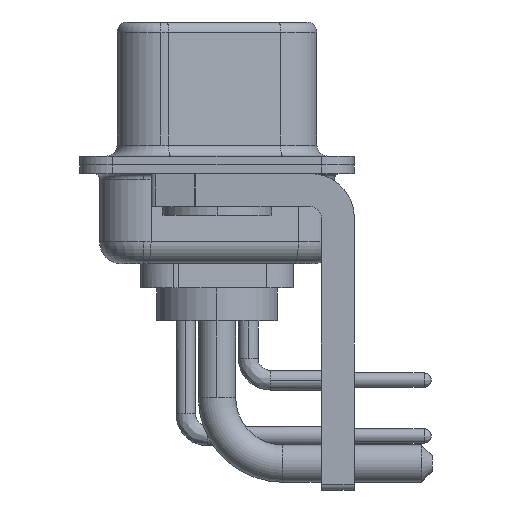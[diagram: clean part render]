
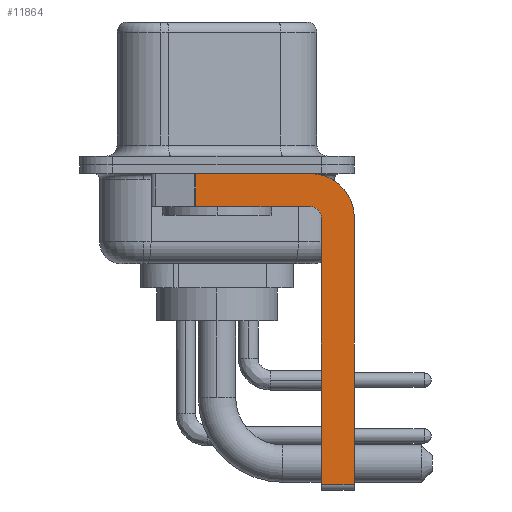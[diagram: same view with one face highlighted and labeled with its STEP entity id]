
A CAD part, left-side view. The second image highlights one B-rep face of the part: STEP entity #11864.
In plain terms, the highlighted planar face has unit normal (-1, 0, 0).
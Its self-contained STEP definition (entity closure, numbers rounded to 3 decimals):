
#256 = EDGE_CURVE ( 'NONE', #3288, #9810, #10729, .T. ) ;
#494 = DIRECTION ( 'NONE',  ( -1., 0., 0. ) ) ;
#2992 = CARTESIAN_POINT ( 'NONE',  ( -2.9, -4.75, -14.55 ) ) ;
#3288 = VERTEX_POINT ( 'NONE', #2992 ) ;
#3813 = CIRCLE ( 'NONE', #5462, 2. ) ;
#4570 = ORIENTED_EDGE ( 'NONE', *, *, #22148, .F. ) ;
#5192 = ORIENTED_EDGE ( 'NONE', *, *, #256, .T. ) ;
#5462 = AXIS2_PLACEMENT_3D ( 'NONE', #16616, #24374, #10972 ) ;
#5881 = ORIENTED_EDGE ( 'NONE', *, *, #9076, .F. ) ;
#6111 = DIRECTION ( 'NONE',  ( 0., 0., 1. ) ) ;
#6135 = DIRECTION ( 'NONE',  ( 0., 0., -1. ) ) ;
#8225 = CARTESIAN_POINT ( 'NONE',  ( -2.9, -4.25, -0.4 ) ) ;
#8263 = ORIENTED_EDGE ( 'NONE', *, *, #18719, .F. ) ;
#8955 = CARTESIAN_POINT ( 'NONE',  ( -2.9, -4.25, -1.9 ) ) ;
#9076 = EDGE_CURVE ( 'NONE', #23849, #9810, #12481, .T. ) ;
#9472 = VECTOR ( 'NONE', #22006, 1000. ) ;
#9617 = VECTOR ( 'NONE', #11481, 1000. ) ;
#9810 = VERTEX_POINT ( 'NONE', #19464 ) ;
#9911 = VERTEX_POINT ( 'NONE', #8225 ) ;
#10006 = LINE ( 'NONE', #13961, #9472 ) ;
#10729 = LINE ( 'NONE', #16484, #17761 ) ;
#10972 = DIRECTION ( 'NONE',  ( 0., 0., -1. ) ) ;
#11234 = VERTEX_POINT ( 'NONE', #13972 ) ;
#11481 = DIRECTION ( 'NONE',  ( 0., 0., 1. ) ) ;
#11592 = CARTESIAN_POINT ( 'NONE',  ( -2.9, -6.25, -2.4 ) ) ;
#11864 = ADVANCED_FACE ( 'NONE', ( #23629 ), #12280, .F. ) ;
#12131 = CARTESIAN_POINT ( 'NONE',  ( -2.9, -4.25, -1.9 ) ) ;
#12280 = PLANE ( 'NONE',  #19416 ) ;
#12481 = LINE ( 'NONE', #18124, #17332 ) ;
#12511 = CARTESIAN_POINT ( 'NONE',  ( -2.9, -4.75, -2.4 ) ) ;
#12883 = VECTOR ( 'NONE', #15212, 1000. ) ;
#13308 = LINE ( 'NONE', #21090, #19061 ) ;
#13311 = ORIENTED_EDGE ( 'NONE', *, *, #20724, .F. ) ;
#13601 = ORIENTED_EDGE ( 'NONE', *, *, #15613, .T. ) ;
#13652 = LINE ( 'NONE', #19516, #9617 ) ;
#13961 = CARTESIAN_POINT ( 'NONE',  ( -2.9, 0.978, -1.9 ) ) ;
#13972 = CARTESIAN_POINT ( 'NONE',  ( -2.9, 0.978, -0.4 ) ) ;
#14074 = CARTESIAN_POINT ( 'NONE',  ( -2.9, -4.25, -2.4 ) ) ;
#14268 = VERTEX_POINT ( 'NONE', #18053 ) ;
#14356 = CIRCLE ( 'NONE', #19639, 0.5 ) ;
#14729 = VERTEX_POINT ( 'NONE', #12131 ) ;
#14732 = EDGE_CURVE ( 'NONE', #19097, #14729, #14356, .T. ) ;
#15212 = DIRECTION ( 'NONE',  ( 0., 1., 0. ) ) ;
#15613 = EDGE_CURVE ( 'NONE', #11234, #14268, #10006, .T. ) ;
#16484 = CARTESIAN_POINT ( 'NONE',  ( -2.9, -4.25, -14.55 ) ) ;
#16616 = CARTESIAN_POINT ( 'NONE',  ( -2.9, -4.25, -2.4 ) ) ;
#17332 = VECTOR ( 'NONE', #17389, 1000. ) ;
#17389 = DIRECTION ( 'NONE',  ( 0., 0., -1. ) ) ;
#17485 = EDGE_CURVE ( 'NONE', #9911, #23849, #3813, .T. ) ;
#17761 = VECTOR ( 'NONE', #18771, 1000. ) ;
#18022 = CARTESIAN_POINT ( 'NONE',  ( -2.9, -4.25, -2.4 ) ) ;
#18053 = CARTESIAN_POINT ( 'NONE',  ( -2.9, 0.978, -1.9 ) ) ;
#18124 = CARTESIAN_POINT ( 'NONE',  ( -2.9, -6.25, -2.4 ) ) ;
#18719 = EDGE_CURVE ( 'NONE', #14729, #14268, #22862, .T. ) ;
#18771 = DIRECTION ( 'NONE',  ( 0., -1., 0. ) ) ;
#19061 = VECTOR ( 'NONE', #20288, 1000. ) ;
#19097 = VERTEX_POINT ( 'NONE', #12511 ) ;
#19273 = EDGE_LOOP ( 'NONE', ( #4570, #13601, #8263, #25105, #13311, #5192, #5881, #23931 ) ) ;
#19416 = AXIS2_PLACEMENT_3D ( 'NONE', #14074, #21864, #6135 ) ;
#19464 = CARTESIAN_POINT ( 'NONE',  ( -2.9, -6.25, -14.55 ) ) ;
#19516 = CARTESIAN_POINT ( 'NONE',  ( -2.9, -4.75, -14.8 ) ) ;
#19639 = AXIS2_PLACEMENT_3D ( 'NONE', #18022, #494, #6111 ) ;
#20288 = DIRECTION ( 'NONE',  ( 0., -1., 0. ) ) ;
#20724 = EDGE_CURVE ( 'NONE', #3288, #19097, #13652, .T. ) ;
#21090 = CARTESIAN_POINT ( 'NONE',  ( -2.9, 3., -0.4 ) ) ;
#21864 = DIRECTION ( 'NONE',  ( 1., 0., 0. ) ) ;
#22006 = DIRECTION ( 'NONE',  ( 0., 0., -1. ) ) ;
#22148 = EDGE_CURVE ( 'NONE', #11234, #9911, #13308, .T. ) ;
#22862 = LINE ( 'NONE', #8955, #12883 ) ;
#23629 = FACE_OUTER_BOUND ( 'NONE', #19273, .T. ) ;
#23849 = VERTEX_POINT ( 'NONE', #11592 ) ;
#23931 = ORIENTED_EDGE ( 'NONE', *, *, #17485, .F. ) ;
#24374 = DIRECTION ( 'NONE',  ( 1., 0., 0. ) ) ;
#25105 = ORIENTED_EDGE ( 'NONE', *, *, #14732, .F. ) ;
